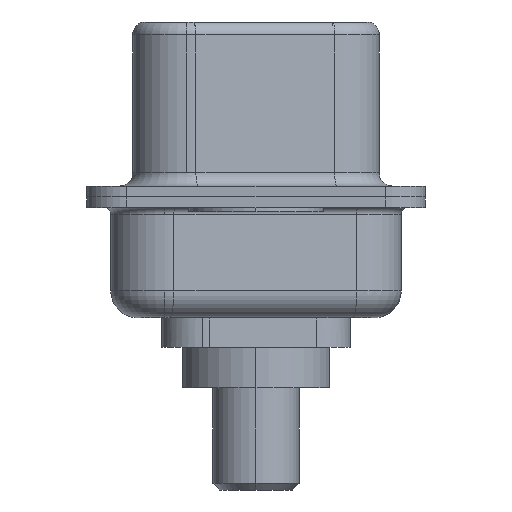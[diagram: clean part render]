
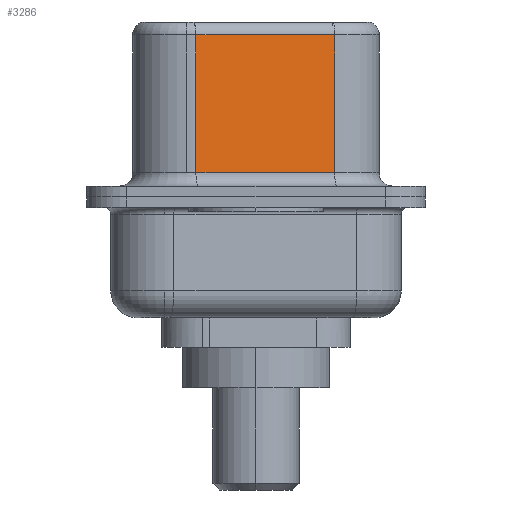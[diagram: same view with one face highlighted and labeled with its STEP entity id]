
A CAD part, left-side view. The second image highlights one B-rep face of the part: STEP entity #3286.
In plain terms, the highlighted planar face has unit normal (-0.985, -0.174, 0).
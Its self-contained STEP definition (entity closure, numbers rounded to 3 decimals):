
#41 = EDGE_CURVE ( 'NONE', #7829, #9919, #2983, .T. ) ;
#329 = LINE ( 'NONE', #2460, #8032 ) ;
#600 = LINE ( 'NONE', #754, #12397 ) ;
#754 = CARTESIAN_POINT ( 'NONE',  ( 4.58, -2.927, 6.02 ) ) ;
#1631 = ORIENTED_EDGE ( 'NONE', *, *, #2109, .F. ) ;
#2086 = CARTESIAN_POINT ( 'NONE',  ( 4.58, -2.927, 0.9 ) ) ;
#2109 = EDGE_CURVE ( 'NONE', #12167, #9919, #7219, .T. ) ;
#2460 = CARTESIAN_POINT ( 'NONE',  ( 3.67, 2.233, 6.52 ) ) ;
#2983 = LINE ( 'NONE', #2086, #6760 ) ;
#3151 = ORIENTED_EDGE ( 'NONE', *, *, #41, .T. ) ;
#3286 = ADVANCED_FACE ( 'NONE', ( #10452 ), #9924, .F. ) ;
#3296 = DIRECTION ( 'NONE',  ( -0.174, 0.985, 0. ) ) ;
#4210 = CARTESIAN_POINT ( 'NONE',  ( 4.58, -2.927, 6.52 ) ) ;
#4706 = CARTESIAN_POINT ( 'NONE',  ( 4.58, -2.927, 0.9 ) ) ;
#5292 = EDGE_CURVE ( 'NONE', #10858, #7829, #329, .T. ) ;
#5477 = VECTOR ( 'NONE', #9651, 1000. ) ;
#5485 = DIRECTION ( 'NONE',  ( 0.985, 0.174, 0. ) ) ;
#5844 = EDGE_LOOP ( 'NONE', ( #1631, #6659, #8203, #3151 ) ) ;
#5979 = CARTESIAN_POINT ( 'NONE',  ( 3.67, 2.233, 6.02 ) ) ;
#6659 = ORIENTED_EDGE ( 'NONE', *, *, #12974, .T. ) ;
#6760 = VECTOR ( 'NONE', #8803, 1000. ) ;
#7217 = AXIS2_PLACEMENT_3D ( 'NONE', #10065, #5485, #3296 ) ;
#7219 = LINE ( 'NONE', #4210, #5477 ) ;
#7829 = VERTEX_POINT ( 'NONE', #11450 ) ;
#8032 = VECTOR ( 'NONE', #12221, 1000. ) ;
#8203 = ORIENTED_EDGE ( 'NONE', *, *, #5292, .T. ) ;
#8589 = DIRECTION ( 'NONE',  ( -0.174, 0.985, 0. ) ) ;
#8803 = DIRECTION ( 'NONE',  ( 0.174, -0.985, 0. ) ) ;
#9651 = DIRECTION ( 'NONE',  ( 0., 0., -1. ) ) ;
#9919 = VERTEX_POINT ( 'NONE', #4706 ) ;
#9924 = PLANE ( 'NONE',  #7217 ) ;
#10065 = CARTESIAN_POINT ( 'NONE',  ( 4.58, -2.927, 6.52 ) ) ;
#10452 = FACE_OUTER_BOUND ( 'NONE', #5844, .T. ) ;
#10858 = VERTEX_POINT ( 'NONE', #5979 ) ;
#11450 = CARTESIAN_POINT ( 'NONE',  ( 3.67, 2.233, 0.9 ) ) ;
#12167 = VERTEX_POINT ( 'NONE', #14078 ) ;
#12221 = DIRECTION ( 'NONE',  ( 0., 0., -1. ) ) ;
#12397 = VECTOR ( 'NONE', #8589, 1000. ) ;
#12974 = EDGE_CURVE ( 'NONE', #12167, #10858, #600, .T. ) ;
#14078 = CARTESIAN_POINT ( 'NONE',  ( 4.58, -2.927, 6.02 ) ) ;
